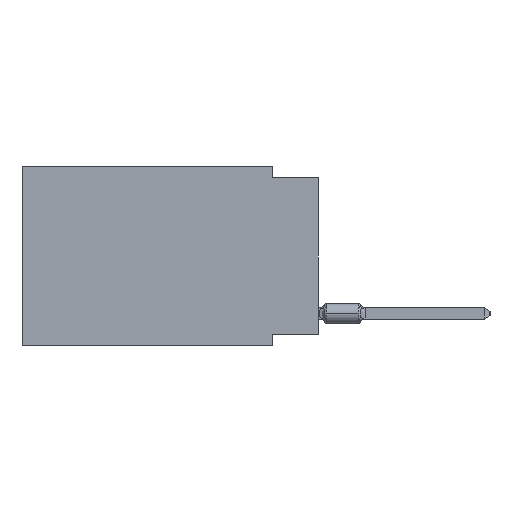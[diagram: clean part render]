
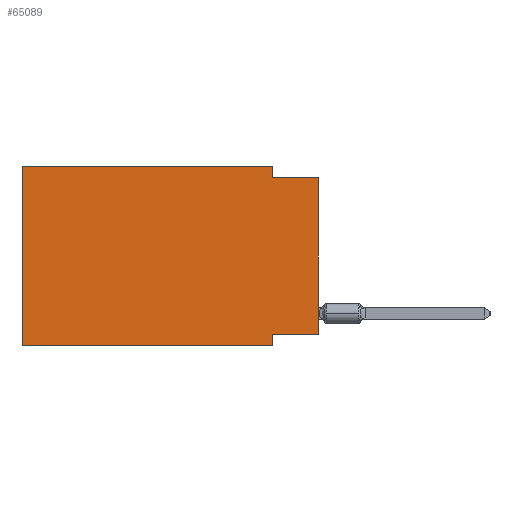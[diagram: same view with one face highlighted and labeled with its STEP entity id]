
A CAD part, left-side view. The second image highlights one B-rep face of the part: STEP entity #65089.
In plain terms, the highlighted planar face has unit normal (-1, 0, 0).
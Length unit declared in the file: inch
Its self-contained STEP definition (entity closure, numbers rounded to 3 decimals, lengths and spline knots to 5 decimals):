
#1818 = VECTOR ( 'NONE', #8536, 39.37008 ) ;
#3027 = CARTESIAN_POINT ( 'NONE',  ( 0., 0.1, -0.025 ) ) ;
#3553 = CARTESIAN_POINT ( 'NONE',  ( 0., 0.1, 0. ) ) ;
#3986 = DIRECTION ( 'NONE',  ( 0., -1., 0. ) ) ;
#4862 = VERTEX_POINT ( 'NONE', #3553 ) ;
#5786 = LINE ( 'NONE', #46329, #82246 ) ;
#6824 = CARTESIAN_POINT ( 'NONE',  ( 0., 0.645, -0.39 ) ) ;
#6923 = ORIENTED_EDGE ( 'NONE', *, *, #31055, .F. ) ;
#8536 = DIRECTION ( 'NONE',  ( 0., 0., -1. ) ) ;
#9913 = FACE_OUTER_BOUND ( 'NONE', #35830, .T. ) ;
#12597 = AXIS2_PLACEMENT_3D ( 'NONE', #23294, #70949, #37499 ) ;
#17432 = VERTEX_POINT ( 'NONE', #27560 ) ;
#17586 = VERTEX_POINT ( 'NONE', #18500 ) ;
#18500 = CARTESIAN_POINT ( 'NONE',  ( 0., 0.645, -0.39 ) ) ;
#18579 = DIRECTION ( 'NONE',  ( 0., 0., 1. ) ) ;
#19428 = CARTESIAN_POINT ( 'NONE',  ( 0., 0., 0. ) ) ;
#22459 = ORIENTED_EDGE ( 'NONE', *, *, #33743, .F. ) ;
#22794 = CARTESIAN_POINT ( 'NONE',  ( 0., 0.1, -0.39 ) ) ;
#23170 = VERTEX_POINT ( 'NONE', #68204 ) ;
#23294 = CARTESIAN_POINT ( 'NONE',  ( 0., 0.645, 0. ) ) ;
#25121 = ORIENTED_EDGE ( 'NONE', *, *, #53259, .F. ) ;
#27560 = CARTESIAN_POINT ( 'NONE',  ( 0., 0.1, -0.39 ) ) ;
#30854 = CARTESIAN_POINT ( 'NONE',  ( 0., 0., -0.365 ) ) ;
#31055 = EDGE_CURVE ( 'NONE', #23170, #49436, #78097, .T. ) ;
#32373 = CARTESIAN_POINT ( 'NONE',  ( 0., 0.645, 0. ) ) ;
#32874 = ORIENTED_EDGE ( 'NONE', *, *, #59566, .T. ) ;
#33223 = DIRECTION ( 'NONE',  ( 0., 0., 1. ) ) ;
#33743 = EDGE_CURVE ( 'NONE', #75117, #74321, #48308, .T. ) ;
#34934 = DIRECTION ( 'NONE',  ( 0., -1., 0. ) ) ;
#35830 = EDGE_LOOP ( 'NONE', ( #49369, #22459, #77632, #58463, #43186, #32874, #25121, #6923 ) ) ;
#37499 = DIRECTION ( 'NONE',  ( 0., 0., -1. ) ) ;
#39456 = EDGE_CURVE ( 'NONE', #17586, #41077, #66258, .T. ) ;
#40761 = VECTOR ( 'NONE', #3986, 39.37008 ) ;
#41077 = VERTEX_POINT ( 'NONE', #53506 ) ;
#42817 = LINE ( 'NONE', #22794, #1818 ) ;
#43186 = ORIENTED_EDGE ( 'NONE', *, *, #39456, .F. ) ;
#43854 = EDGE_CURVE ( 'NONE', #4862, #75117, #5786, .T. ) ;
#46329 = CARTESIAN_POINT ( 'NONE',  ( 0., 0.1, 0. ) ) ;
#48053 = DIRECTION ( 'NONE',  ( 0., 0., -1. ) ) ;
#48308 = LINE ( 'NONE', #75477, #53389 ) ;
#49369 = ORIENTED_EDGE ( 'NONE', *, *, #74908, .T. ) ;
#49436 = VERTEX_POINT ( 'NONE', #66241 ) ;
#53259 = EDGE_CURVE ( 'NONE', #49436, #17432, #42817, .T. ) ;
#53389 = VECTOR ( 'NONE', #34934, 39.37008 ) ;
#53506 = CARTESIAN_POINT ( 'NONE',  ( 0., 0.645, 0. ) ) ;
#54723 = VECTOR ( 'NONE', #58035, 39.37008 ) ;
#58035 = DIRECTION ( 'NONE',  ( 0., 1., 0. ) ) ;
#58463 = ORIENTED_EDGE ( 'NONE', *, *, #62864, .F. ) ;
#59566 = EDGE_CURVE ( 'NONE', #17586, #17432, #87496, .T. ) ;
#62864 = EDGE_CURVE ( 'NONE', #41077, #4862, #85523, .T. ) ;
#65089 = ADVANCED_FACE ( 'NONE', ( #9913 ), #71377, .F. ) ;
#66222 = LINE ( 'NONE', #19428, #81166 ) ;
#66241 = CARTESIAN_POINT ( 'NONE',  ( 0., 0.1, -0.365 ) ) ;
#66258 = LINE ( 'NONE', #32373, #66694 ) ;
#66694 = VECTOR ( 'NONE', #18579, 39.37008 ) ;
#68204 = CARTESIAN_POINT ( 'NONE',  ( 0., 0., -0.365 ) ) ;
#70949 = DIRECTION ( 'NONE',  ( 1., 0., 0. ) ) ;
#71377 = PLANE ( 'NONE',  #12597 ) ;
#71875 = VECTOR ( 'NONE', #74971, 39.37008 ) ;
#74321 = VERTEX_POINT ( 'NONE', #82853 ) ;
#74908 = EDGE_CURVE ( 'NONE', #23170, #74321, #66222, .T. ) ;
#74971 = DIRECTION ( 'NONE',  ( 0., -1., 0. ) ) ;
#75117 = VERTEX_POINT ( 'NONE', #3027 ) ;
#75477 = CARTESIAN_POINT ( 'NONE',  ( 0., 0., -0.025 ) ) ;
#77632 = ORIENTED_EDGE ( 'NONE', *, *, #43854, .F. ) ;
#78097 = LINE ( 'NONE', #30854, #54723 ) ;
#78402 = CARTESIAN_POINT ( 'NONE',  ( 0., 0.645, 0. ) ) ;
#81166 = VECTOR ( 'NONE', #33223, 39.37008 ) ;
#82246 = VECTOR ( 'NONE', #48053, 39.37008 ) ;
#82853 = CARTESIAN_POINT ( 'NONE',  ( 0., 0., -0.025 ) ) ;
#85523 = LINE ( 'NONE', #78402, #40761 ) ;
#87496 = LINE ( 'NONE', #6824, #71875 ) ;
